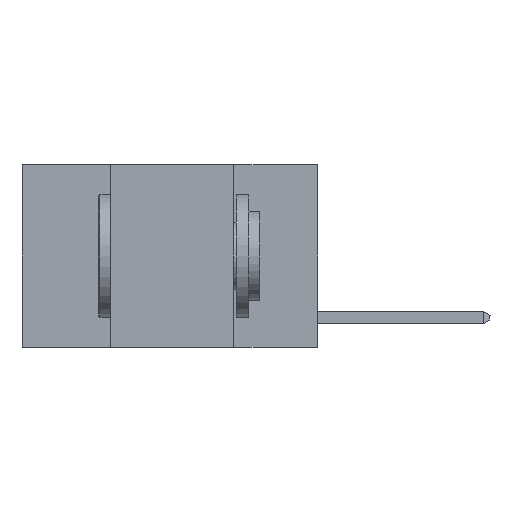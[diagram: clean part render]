
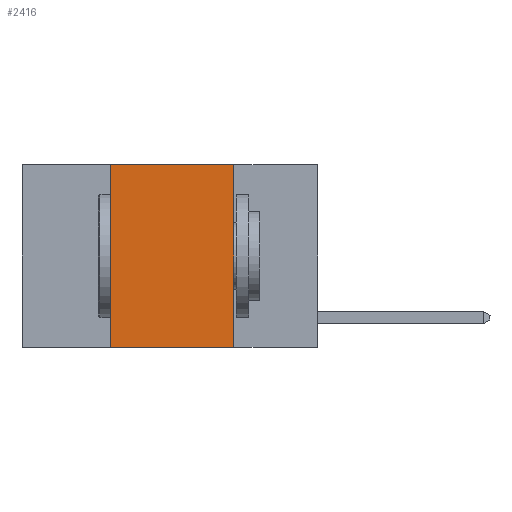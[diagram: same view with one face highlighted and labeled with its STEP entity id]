
A CAD part, left-side view. The second image highlights one B-rep face of the part: STEP entity #2416.
In plain terms, the highlighted planar face has unit normal (-1, 0, 0).
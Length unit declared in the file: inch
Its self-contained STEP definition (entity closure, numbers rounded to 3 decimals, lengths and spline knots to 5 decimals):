
#147 = CARTESIAN_POINT ( 'NONE',  ( 0., 0.42, 0. ) ) ;
#247 = EDGE_CURVE ( 'NONE', #13782, #15827, #19758, .T. ) ;
#1059 = PLANE ( 'NONE',  #3732 ) ;
#1959 = EDGE_LOOP ( 'NONE', ( #26297, #12280, #18400, #22942 ) ) ;
#2012 = EDGE_CURVE ( 'NONE', #15827, #4766, #15419, .T. ) ;
#2374 = CARTESIAN_POINT ( 'NONE',  ( 0., 0.17, 0. ) ) ;
#2416 = ADVANCED_FACE ( 'NONE', ( #2779 ), #1059, .F. ) ;
#2779 = FACE_OUTER_BOUND ( 'NONE', #1959, .T. ) ;
#3732 = AXIS2_PLACEMENT_3D ( 'NONE', #13936, #26651, #14069 ) ;
#4766 = VERTEX_POINT ( 'NONE', #2374 ) ;
#5052 = LINE ( 'NONE', #25062, #5793 ) ;
#5793 = VECTOR ( 'NONE', #25210, 39.37008 ) ;
#5913 = LINE ( 'NONE', #10228, #13821 ) ;
#8579 = VERTEX_POINT ( 'NONE', #22226 ) ;
#8873 = DIRECTION ( 'NONE',  ( 0., 0., 1. ) ) ;
#10228 = CARTESIAN_POINT ( 'NONE',  ( 0., 0.17, 0. ) ) ;
#12280 = ORIENTED_EDGE ( 'NONE', *, *, #2012, .F. ) ;
#13782 = VERTEX_POINT ( 'NONE', #20944 ) ;
#13821 = VECTOR ( 'NONE', #14665, 39.37008 ) ;
#13888 = EDGE_CURVE ( 'NONE', #4766, #8579, #5913, .T. ) ;
#13936 = CARTESIAN_POINT ( 'NONE',  ( 0., 0.6, 0. ) ) ;
#14069 = DIRECTION ( 'NONE',  ( 0., 0., -1. ) ) ;
#14665 = DIRECTION ( 'NONE',  ( 0., 0., -1. ) ) ;
#15419 = LINE ( 'NONE', #19867, #16496 ) ;
#15827 = VERTEX_POINT ( 'NONE', #21495 ) ;
#16496 = VECTOR ( 'NONE', #26984, 39.37008 ) ;
#17728 = VECTOR ( 'NONE', #8873, 39.37008 ) ;
#18400 = ORIENTED_EDGE ( 'NONE', *, *, #247, .F. ) ;
#19758 = LINE ( 'NONE', #147, #17728 ) ;
#19867 = CARTESIAN_POINT ( 'NONE',  ( 0., 0.6, 0. ) ) ;
#20944 = CARTESIAN_POINT ( 'NONE',  ( 0., 0.42, -0.37 ) ) ;
#21495 = CARTESIAN_POINT ( 'NONE',  ( 0., 0.42, 0. ) ) ;
#22226 = CARTESIAN_POINT ( 'NONE',  ( 0., 0.17, -0.37 ) ) ;
#22942 = ORIENTED_EDGE ( 'NONE', *, *, #26968, .T. ) ;
#25062 = CARTESIAN_POINT ( 'NONE',  ( 0., 0.6, -0.37 ) ) ;
#25210 = DIRECTION ( 'NONE',  ( 0., -1., 0. ) ) ;
#26297 = ORIENTED_EDGE ( 'NONE', *, *, #13888, .F. ) ;
#26651 = DIRECTION ( 'NONE',  ( 1., 0., 0. ) ) ;
#26968 = EDGE_CURVE ( 'NONE', #13782, #8579, #5052, .T. ) ;
#26984 = DIRECTION ( 'NONE',  ( 0., -1., 0. ) ) ;
